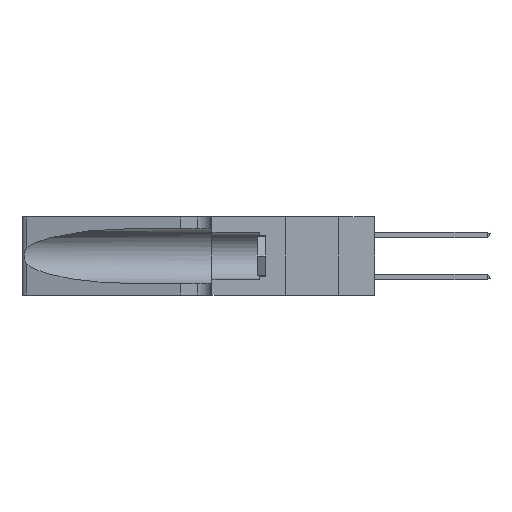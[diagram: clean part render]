
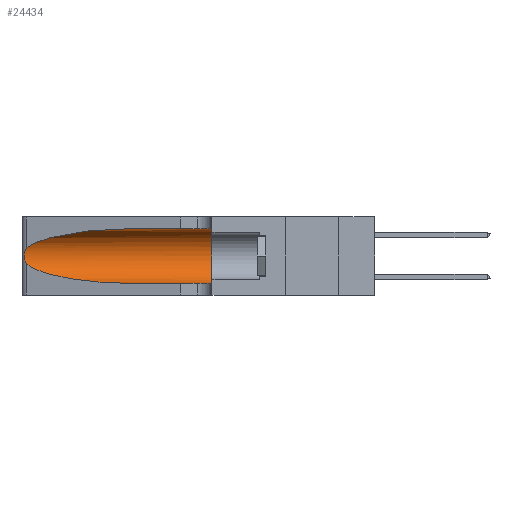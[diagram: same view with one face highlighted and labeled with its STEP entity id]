
A CAD part, left-side view. The second image highlights one B-rep face of the part: STEP entity #24434.
In plain terms, the highlighted cylindrical face has radius 3.308 mm (diameter 6.617 mm), a partial arc.
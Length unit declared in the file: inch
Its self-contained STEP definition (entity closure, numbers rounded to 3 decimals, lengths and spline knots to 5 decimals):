
#265 = CARTESIAN_POINT ( 'NONE',  ( 0.1305, 1.61858, 0.185 ) ) ;
#745 = DIRECTION ( 'NONE',  ( 0., 0., 1. ) ) ;
#1553 = CARTESIAN_POINT ( 'NONE',  ( 0.25789, 1.23486, 0.15765 ) ) ;
#1730 = FACE_OUTER_BOUND ( 'NONE', #3669, .T. ) ;
#2206 = CARTESIAN_POINT ( 'NONE',  ( 0.2373, 1.15595, 0.28018 ) ) ;
#2220 = EDGE_CURVE ( 'NONE', #3901, #6728, #11747, .T. ) ;
#2449 = CARTESIAN_POINT ( 'NONE',  ( 0.25487, 1.22718, 0.22369 ) ) ;
#2733 = VERTEX_POINT ( 'NONE', #13327 ) ;
#3064 = DIRECTION ( 'NONE',  ( 0., -1., 0. ) ) ;
#3669 = EDGE_LOOP ( 'NONE', ( #31855, #14437, #33962, #4222, #19544, #8221 ) ) ;
#3901 = VERTEX_POINT ( 'NONE', #22989 ) ;
#4085 = CARTESIAN_POINT ( 'NONE',  ( 0.25555, 1.22994, 0.2215 ) ) ;
#4222 = ORIENTED_EDGE ( 'NONE', *, *, #29029, .T. ) ;
#4319 = CARTESIAN_POINT ( 'NONE',  ( 0.25555, 1.22993, 0.14849 ) ) ;
#6728 = VERTEX_POINT ( 'NONE', #8726 ) ;
#6976 = AXIS2_PLACEMENT_3D ( 'NONE', #32156, #16771, #745 ) ;
#7682 = CARTESIAN_POINT ( 'NONE',  ( 0.25487, 1.22718, 0.22369 ) ) ;
#8221 = ORIENTED_EDGE ( 'NONE', *, *, #11714, .F. ) ;
#8726 = CARTESIAN_POINT ( 'NONE',  ( 0.1305, 0.35, 0.05475 ) ) ;
#8984 = EDGE_CURVE ( 'NONE', #16779, #30397, #10554, .T. ) ;
#9600 = CARTESIAN_POINT ( 'NONE',  ( 0.25787, 1.23484, 0.2124 ) ) ;
#10554 =( BOUNDED_CURVE ( )  B_SPLINE_CURVE ( 3, ( #23301, #20721, #2206, #7682 ),
 .UNSPECIFIED., .F., .F. ) 
 B_SPLINE_CURVE_WITH_KNOTS ( ( 4, 4 ),
 ( 1.5708, 2.84003 ),
 .UNSPECIFIED. ) 
 CURVE ( )  GEOMETRIC_REPRESENTATION_ITEM ( )  RATIONAL_B_SPLINE_CURVE ( ( 1., 0.87, 0.87, 1. ) ) 
 REPRESENTATION_ITEM ( '' )  );
#11714 = EDGE_CURVE ( 'NONE', #16779, #3901, #29657, .T. ) ;
#11747 = CIRCLE ( 'NONE', #6976, 0.13025 ) ;
#12266 = CARTESIAN_POINT ( 'NONE',  ( 0.26018, 1.23835, 0.19895 ) ) ;
#13327 = CARTESIAN_POINT ( 'NONE',  ( 0.1305, 0.72297, 0.05475 ) ) ;
#14150 =( BOUNDED_CURVE ( )  B_SPLINE_CURVE ( 3, ( #28006, #22858, #33185, #17822 ),
 .UNSPECIFIED., .F., .F. ) 
 B_SPLINE_CURVE_WITH_KNOTS ( ( 4, 4 ),
 ( 3.44316, 4.71239 ),
 .UNSPECIFIED. ) 
 CURVE ( )  GEOMETRIC_REPRESENTATION_ITEM ( )  RATIONAL_B_SPLINE_CURVE ( ( 1., 0.87, 0.87, 1. ) ) 
 REPRESENTATION_ITEM ( '' )  );
#14437 = ORIENTED_EDGE ( 'NONE', *, *, #16271, .T. ) ;
#14927 = CARTESIAN_POINT ( 'NONE',  ( 0.26075, 1.23896, 0.178 ) ) ;
#15153 = CYLINDRICAL_SURFACE ( 'NONE', #15233, 0.13025 ) ;
#15233 = AXIS2_PLACEMENT_3D ( 'NONE', #265, #3064, #16336 ) ;
#15383 = CARTESIAN_POINT ( 'NONE',  ( 0.1305, 1.61858, 0.05475 ) ) ;
#16271 = EDGE_CURVE ( 'NONE', #30397, #30119, #32098, .T. ) ;
#16336 = DIRECTION ( 'NONE',  ( 0., 0., -1. ) ) ;
#16771 = DIRECTION ( 'NONE',  ( 0., 1., 0. ) ) ;
#16779 = VERTEX_POINT ( 'NONE', #32307 ) ;
#16786 = VECTOR ( 'NONE', #18677, 39.37008 ) ;
#17562 = CARTESIAN_POINT ( 'NONE',  ( 0.25856, 1.23593, 0.16098 ) ) ;
#17822 = CARTESIAN_POINT ( 'NONE',  ( 0.1305, 0.72297, 0.05475 ) ) ;
#18677 = DIRECTION ( 'NONE',  ( 0., -1., 0. ) ) ;
#19544 = ORIENTED_EDGE ( 'NONE', *, *, #2220, .F. ) ;
#20132 = CARTESIAN_POINT ( 'NONE',  ( 0.25639, 1.23186, 0.15144 ) ) ;
#20721 = CARTESIAN_POINT ( 'NONE',  ( 0.18966, 0.96281, 0.31525 ) ) ;
#21726 = VECTOR ( 'NONE', #23048, 39.37008 ) ;
#22396 = CARTESIAN_POINT ( 'NONE',  ( 0.25487, 1.22718, 0.14631 ) ) ;
#22704 = CARTESIAN_POINT ( 'NONE',  ( 0.25487, 1.22718, 0.14631 ) ) ;
#22858 = CARTESIAN_POINT ( 'NONE',  ( 0.2373, 1.15595, 0.08982 ) ) ;
#22989 = CARTESIAN_POINT ( 'NONE',  ( 0.1305, 0.35, 0.31525 ) ) ;
#23048 = DIRECTION ( 'NONE',  ( 0., -1., 0. ) ) ;
#23301 = CARTESIAN_POINT ( 'NONE',  ( 0.1305, 0.72297, 0.31525 ) ) ;
#23343 = LINE ( 'NONE', #15383, #21726 ) ;
#24434 = ADVANCED_FACE ( 'NONE', ( #1730 ), #15153, .F. ) ;
#24787 = EDGE_CURVE ( 'NONE', #30119, #2733, #14150, .T. ) ;
#25172 = CARTESIAN_POINT ( 'NONE',  ( 0.25639, 1.23184, 0.21858 ) ) ;
#27756 = CARTESIAN_POINT ( 'NONE',  ( 0.25854, 1.2359, 0.20912 ) ) ;
#28006 = CARTESIAN_POINT ( 'NONE',  ( 0.25487, 1.22718, 0.14631 ) ) ;
#29029 = EDGE_CURVE ( 'NONE', #2733, #6728, #23343, .T. ) ;
#29657 = LINE ( 'NONE', #31465, #16786 ) ;
#30119 = VERTEX_POINT ( 'NONE', #22396 ) ;
#30348 = CARTESIAN_POINT ( 'NONE',  ( 0.26075, 1.23896, 0.19203 ) ) ;
#30397 = VERTEX_POINT ( 'NONE', #2449 ) ;
#31465 = CARTESIAN_POINT ( 'NONE',  ( 0.1305, 1.61858, 0.31525 ) ) ;
#31855 = ORIENTED_EDGE ( 'NONE', *, *, #8984, .T. ) ;
#32098 = B_SPLINE_CURVE_WITH_KNOTS ( 'NONE', 3,
 ( #32806, #4085, #25172, #9600, #27756, #12266, #30348, #14927, #32919, #17562, #1553, #20132, #4319, #22704 ),
 .UNSPECIFIED., .F., .F.,
 ( 4, 2, 2, 2, 2, 2, 4 ),
 ( 0., 0.00027, 0.00053, 0.00107, 0.0016, 0.00187, 0.00214 ),
 .UNSPECIFIED. ) ;
#32156 = CARTESIAN_POINT ( 'NONE',  ( 0.1305, 0.35, 0.185 ) ) ;
#32307 = CARTESIAN_POINT ( 'NONE',  ( 0.1305, 0.72297, 0.31525 ) ) ;
#32806 = CARTESIAN_POINT ( 'NONE',  ( 0.25487, 1.22718, 0.22369 ) ) ;
#32919 = CARTESIAN_POINT ( 'NONE',  ( 0.26017, 1.23833, 0.17102 ) ) ;
#33185 = CARTESIAN_POINT ( 'NONE',  ( 0.18966, 0.96281, 0.05475 ) ) ;
#33962 = ORIENTED_EDGE ( 'NONE', *, *, #24787, .T. ) ;
